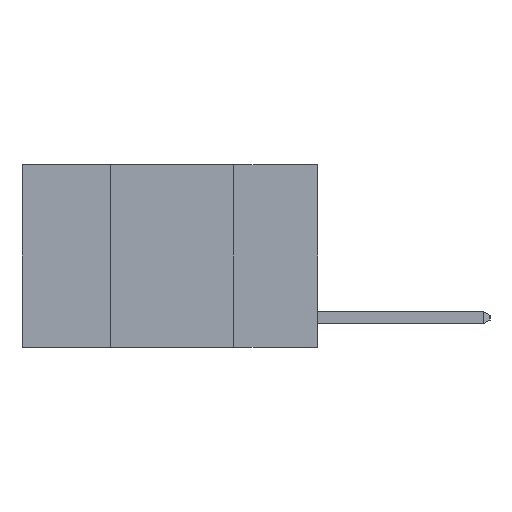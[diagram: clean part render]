
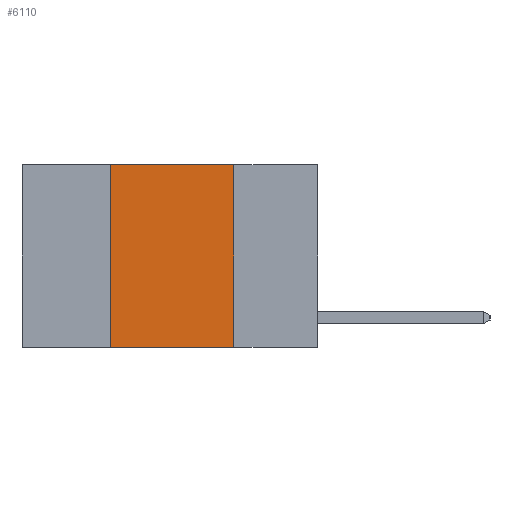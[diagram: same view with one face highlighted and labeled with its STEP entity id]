
A CAD part, left-side view. The second image highlights one B-rep face of the part: STEP entity #6110.
In plain terms, the highlighted planar face has unit normal (-1, 0, 0).
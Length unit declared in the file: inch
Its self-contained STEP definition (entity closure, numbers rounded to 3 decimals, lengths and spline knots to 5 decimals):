
#239 = VERTEX_POINT ( 'NONE', #7779 ) ;
#240 = EDGE_CURVE ( 'NONE', #6784, #239, #3070, .T. ) ;
#242 = DIRECTION ( 'NONE',  ( 0., 0., -1. ) ) ;
#501 = CARTESIAN_POINT ( 'NONE',  ( 0., 0.17, 0. ) ) ;
#1068 = DIRECTION ( 'NONE',  ( 0., 0., 1. ) ) ;
#1246 = CARTESIAN_POINT ( 'NONE',  ( 0., 0.42, 0. ) ) ;
#1345 = VECTOR ( 'NONE', #3244, 39.37008 ) ;
#1638 = CARTESIAN_POINT ( 'NONE',  ( 0., 0.6, 0. ) ) ;
#1773 = ORIENTED_EDGE ( 'NONE', *, *, #240, .F. ) ;
#1917 = LINE ( 'NONE', #2714, #3592 ) ;
#2196 = EDGE_CURVE ( 'NONE', #5533, #7047, #7449, .T. ) ;
#2519 = CARTESIAN_POINT ( 'NONE',  ( 0., 0.6, -0.37 ) ) ;
#2714 = CARTESIAN_POINT ( 'NONE',  ( 0., 0.6, 0. ) ) ;
#2925 = FACE_OUTER_BOUND ( 'NONE', #4043, .T. ) ;
#3070 = LINE ( 'NONE', #501, #8489 ) ;
#3244 = DIRECTION ( 'NONE',  ( 0., -1., 0. ) ) ;
#3369 = ORIENTED_EDGE ( 'NONE', *, *, #6282, .T. ) ;
#3589 = ORIENTED_EDGE ( 'NONE', *, *, #2196, .F. ) ;
#3592 = VECTOR ( 'NONE', #8364, 39.37008 ) ;
#3781 = PLANE ( 'NONE',  #8698 ) ;
#4043 = EDGE_LOOP ( 'NONE', ( #1773, #8769, #3589, #3369 ) ) ;
#4520 = DIRECTION ( 'NONE',  ( 0., 0., -1. ) ) ;
#4733 = CARTESIAN_POINT ( 'NONE',  ( 0., 0.42, 0. ) ) ;
#5189 = CARTESIAN_POINT ( 'NONE',  ( 0., 0.17, 0. ) ) ;
#5533 = VERTEX_POINT ( 'NONE', #6036 ) ;
#6036 = CARTESIAN_POINT ( 'NONE',  ( 0., 0.42, -0.37 ) ) ;
#6110 = ADVANCED_FACE ( 'NONE', ( #2925 ), #3781, .F. ) ;
#6282 = EDGE_CURVE ( 'NONE', #5533, #239, #7215, .T. ) ;
#6418 = EDGE_CURVE ( 'NONE', #7047, #6784, #1917, .T. ) ;
#6784 = VERTEX_POINT ( 'NONE', #5189 ) ;
#7047 = VERTEX_POINT ( 'NONE', #4733 ) ;
#7213 = VECTOR ( 'NONE', #1068, 39.37008 ) ;
#7215 = LINE ( 'NONE', #2519, #1345 ) ;
#7449 = LINE ( 'NONE', #1246, #7213 ) ;
#7779 = CARTESIAN_POINT ( 'NONE',  ( 0., 0.17, -0.37 ) ) ;
#8364 = DIRECTION ( 'NONE',  ( 0., -1., 0. ) ) ;
#8489 = VECTOR ( 'NONE', #242, 39.37008 ) ;
#8698 = AXIS2_PLACEMENT_3D ( 'NONE', #1638, #8712, #4520 ) ;
#8712 = DIRECTION ( 'NONE',  ( 1., 0., 0. ) ) ;
#8769 = ORIENTED_EDGE ( 'NONE', *, *, #6418, .F. ) ;
